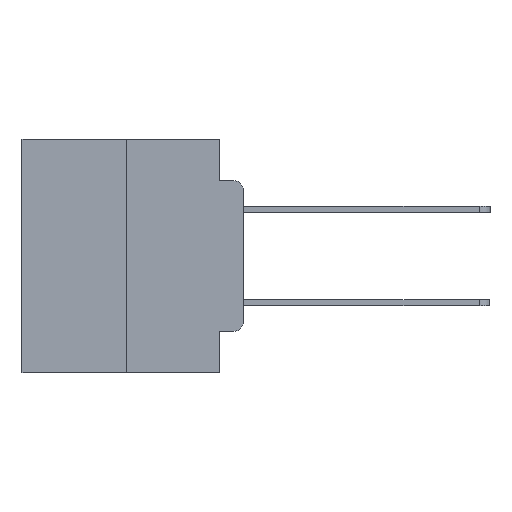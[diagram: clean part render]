
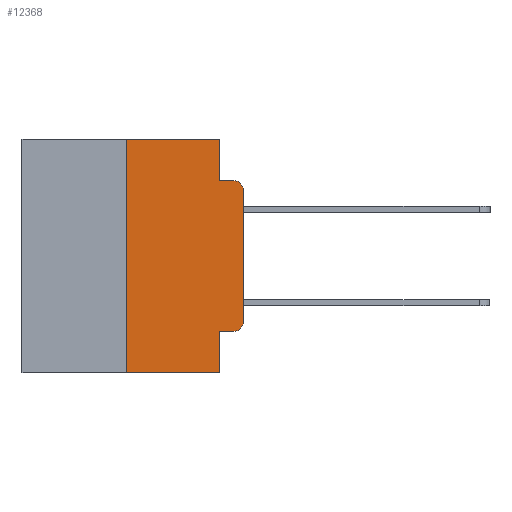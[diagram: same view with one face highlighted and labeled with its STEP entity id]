
A CAD part, left-side view. The second image highlights one B-rep face of the part: STEP entity #12368.
In plain terms, the highlighted planar face has unit normal (-1, 0, 0).
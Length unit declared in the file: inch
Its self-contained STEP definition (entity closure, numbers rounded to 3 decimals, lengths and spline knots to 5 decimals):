
#19 = DIRECTION ( 'NONE',  ( 0., 0., -1. ) ) ;
#46 = ORIENTED_EDGE ( 'NONE', *, *, #4166, .T. ) ;
#474 = LINE ( 'NONE', #14505, #15134 ) ;
#488 = CARTESIAN_POINT ( 'NONE',  ( 0., 0., -0.3915 ) ) ;
#1719 = ORIENTED_EDGE ( 'NONE', *, *, #26309, .T. ) ;
#1941 = ORIENTED_EDGE ( 'NONE', *, *, #8517, .F. ) ;
#2144 = CIRCLE ( 'NONE', #10463, 0.02 ) ;
#2951 = DIRECTION ( 'NONE',  ( 1., 0., 0. ) ) ;
#3591 = DIRECTION ( 'NONE',  ( 0., 0., -1. ) ) ;
#3661 = VERTEX_POINT ( 'NONE', #7345 ) ;
#3703 = ORIENTED_EDGE ( 'NONE', *, *, #12575, .F. ) ;
#4166 = EDGE_CURVE ( 'NONE', #7461, #17594, #474, .T. ) ;
#4411 = VERTEX_POINT ( 'NONE', #15895 ) ;
#4758 = VERTEX_POINT ( 'NONE', #23584 ) ;
#4786 = VECTOR ( 'NONE', #16340, 39.37008 ) ;
#5148 = CARTESIAN_POINT ( 'NONE',  ( 0., 0.051, -0.0885 ) ) ;
#5189 = ORIENTED_EDGE ( 'NONE', *, *, #14834, .T. ) ;
#5408 = VECTOR ( 'NONE', #19607, 39.37008 ) ;
#5999 = CARTESIAN_POINT ( 'NONE',  ( 0., 0.051, 0. ) ) ;
#6345 = VERTEX_POINT ( 'NONE', #488 ) ;
#6444 = LINE ( 'NONE', #5148, #22013 ) ;
#7210 = FACE_OUTER_BOUND ( 'NONE', #7801, .T. ) ;
#7345 = CARTESIAN_POINT ( 'NONE',  ( 0., 0.051, 0. ) ) ;
#7461 = VERTEX_POINT ( 'NONE', #14176 ) ;
#7521 = VECTOR ( 'NONE', #22005, 39.37008 ) ;
#7801 = EDGE_LOOP ( 'NONE', ( #5189, #18280, #1941, #24471, #3703, #17858, #46, #9916, #1719, #18184 ) ) ;
#8004 = VERTEX_POINT ( 'NONE', #9760 ) ;
#8109 = DIRECTION ( 'NONE',  ( 0., 0., -1. ) ) ;
#8341 = LINE ( 'NONE', #5999, #18503 ) ;
#8517 = EDGE_CURVE ( 'NONE', #4411, #4758, #6444, .T. ) ;
#8815 = EDGE_CURVE ( 'NONE', #7461, #22152, #20435, .T. ) ;
#9242 = VECTOR ( 'NONE', #15994, 39.37008 ) ;
#9406 = CARTESIAN_POINT ( 'NONE',  ( 0., 0., 0. ) ) ;
#9708 = DIRECTION ( 'NONE',  ( 0., -1., 0. ) ) ;
#9760 = CARTESIAN_POINT ( 'NONE',  ( 0., 0.051, -0.4115 ) ) ;
#9868 = CARTESIAN_POINT ( 'NONE',  ( 0., 0.473, 0. ) ) ;
#9916 = ORIENTED_EDGE ( 'NONE', *, *, #23601, .F. ) ;
#10463 = AXIS2_PLACEMENT_3D ( 'NONE', #24456, #12371, #26484 ) ;
#10617 = CARTESIAN_POINT ( 'NONE',  ( 0., 0.051, -0.5 ) ) ;
#11914 = VERTEX_POINT ( 'NONE', #20050 ) ;
#11920 = CARTESIAN_POINT ( 'NONE',  ( 0., 0.051, -0.4115 ) ) ;
#12368 = ADVANCED_FACE ( 'NONE', ( #7210 ), #21333, .F. ) ;
#12371 = DIRECTION ( 'NONE',  ( -1., 0., 0. ) ) ;
#12560 = EDGE_CURVE ( 'NONE', #3661, #4411, #18317, .T. ) ;
#12567 = DIRECTION ( 'NONE',  ( -1., 0., 0. ) ) ;
#12575 = EDGE_CURVE ( 'NONE', #22152, #3661, #24310, .T. ) ;
#12771 = EDGE_CURVE ( 'NONE', #11914, #6345, #13259, .T. ) ;
#12942 = VECTOR ( 'NONE', #3591, 39.37008 ) ;
#13194 = CARTESIAN_POINT ( 'NONE',  ( 0., 0.25, 0. ) ) ;
#13198 = EDGE_CURVE ( 'NONE', #13775, #4758, #2144, .T. ) ;
#13259 = CIRCLE ( 'NONE', #19633, 0.02 ) ;
#13775 = VERTEX_POINT ( 'NONE', #16165 ) ;
#14176 = CARTESIAN_POINT ( 'NONE',  ( 0., 0.25, -0.5 ) ) ;
#14505 = CARTESIAN_POINT ( 'NONE',  ( 0., 0.473, -0.5 ) ) ;
#14834 = EDGE_CURVE ( 'NONE', #6345, #13775, #16315, .T. ) ;
#15134 = VECTOR ( 'NONE', #9708, 39.37008 ) ;
#15337 = LINE ( 'NONE', #11920, #9242 ) ;
#15368 = CARTESIAN_POINT ( 'NONE',  ( 0., 0.473, 0. ) ) ;
#15895 = CARTESIAN_POINT ( 'NONE',  ( 0., 0.051, -0.0885 ) ) ;
#15994 = DIRECTION ( 'NONE',  ( 0., -1., 0. ) ) ;
#16165 = CARTESIAN_POINT ( 'NONE',  ( 0., 0., -0.1085 ) ) ;
#16315 = LINE ( 'NONE', #9406, #5408 ) ;
#16340 = DIRECTION ( 'NONE',  ( 0., 0., 1. ) ) ;
#17378 = DIRECTION ( 'NONE',  ( 0., 0., -1. ) ) ;
#17594 = VERTEX_POINT ( 'NONE', #10617 ) ;
#17858 = ORIENTED_EDGE ( 'NONE', *, *, #8815, .F. ) ;
#18184 = ORIENTED_EDGE ( 'NONE', *, *, #12771, .T. ) ;
#18280 = ORIENTED_EDGE ( 'NONE', *, *, #13198, .T. ) ;
#18317 = LINE ( 'NONE', #21922, #12942 ) ;
#18503 = VECTOR ( 'NONE', #8109, 39.37008 ) ;
#18781 = AXIS2_PLACEMENT_3D ( 'NONE', #15368, #2951, #17378 ) ;
#19429 = DIRECTION ( 'NONE',  ( 0., -1., 0. ) ) ;
#19607 = DIRECTION ( 'NONE',  ( 0., 0., 1. ) ) ;
#19633 = AXIS2_PLACEMENT_3D ( 'NONE', #24639, #12567, #19 ) ;
#20050 = CARTESIAN_POINT ( 'NONE',  ( 0., 0.02, -0.4115 ) ) ;
#20435 = LINE ( 'NONE', #26387, #4786 ) ;
#21333 = PLANE ( 'NONE',  #18781 ) ;
#21922 = CARTESIAN_POINT ( 'NONE',  ( 0., 0.051, 0. ) ) ;
#22005 = DIRECTION ( 'NONE',  ( 0., -1., 0. ) ) ;
#22013 = VECTOR ( 'NONE', #19429, 39.37008 ) ;
#22152 = VERTEX_POINT ( 'NONE', #13194 ) ;
#23584 = CARTESIAN_POINT ( 'NONE',  ( 0., 0.02, -0.0885 ) ) ;
#23601 = EDGE_CURVE ( 'NONE', #8004, #17594, #8341, .T. ) ;
#24310 = LINE ( 'NONE', #9868, #7521 ) ;
#24456 = CARTESIAN_POINT ( 'NONE',  ( 0., 0.02, -0.1085 ) ) ;
#24471 = ORIENTED_EDGE ( 'NONE', *, *, #12560, .F. ) ;
#24639 = CARTESIAN_POINT ( 'NONE',  ( 0., 0.02, -0.3915 ) ) ;
#26309 = EDGE_CURVE ( 'NONE', #8004, #11914, #15337, .T. ) ;
#26387 = CARTESIAN_POINT ( 'NONE',  ( 0., 0.25, 0. ) ) ;
#26484 = DIRECTION ( 'NONE',  ( 0., 0., -1. ) ) ;
